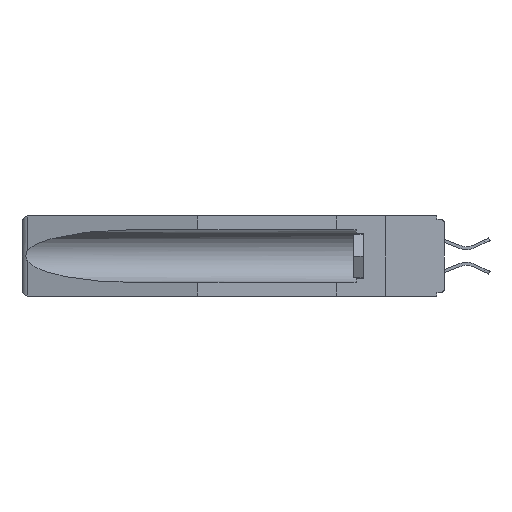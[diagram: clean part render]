
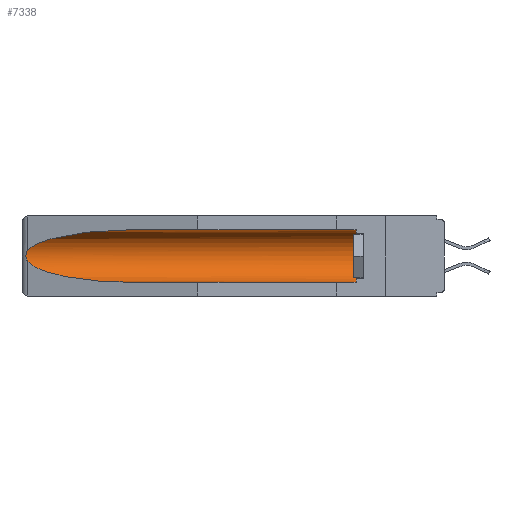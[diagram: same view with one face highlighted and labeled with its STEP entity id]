
A CAD part, left-side view. The second image highlights one B-rep face of the part: STEP entity #7338.
In plain terms, the highlighted cylindrical face has radius 2.857 mm (diameter 5.715 mm), a partial arc.
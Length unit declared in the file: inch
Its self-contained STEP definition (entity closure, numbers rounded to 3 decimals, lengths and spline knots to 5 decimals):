
#56 = LINE ( 'NONE', #18572, #3285 ) ;
#60 = VERTEX_POINT ( 'NONE', #5530 ) ;
#627 = CARTESIAN_POINT ( 'NONE',  ( 0.26537, 1.52718, -0.19328 ) ) ;
#796 = CARTESIAN_POINT ( 'NONE',  ( 0.155, 0.126, -0.1715 ) ) ;
#917 = DIRECTION ( 'NONE',  ( 0., -1., 0. ) ) ;
#1253 = DIRECTION ( 'NONE',  ( 0., 1., 0. ) ) ;
#1864 = EDGE_CURVE ( 'NONE', #13135, #60, #2921, .T. ) ;
#2001 = CARTESIAN_POINT ( 'NONE',  ( 0.26537, 1.52718, -0.19328 ) ) ;
#2046 = CARTESIAN_POINT ( 'NONE',  ( 0.26654, 1.53092, -0.15636 ) ) ;
#2112 = CARTESIAN_POINT ( 'NONE',  ( 0.2675, 1.53308, -0.16763 ) ) ;
#2241 = EDGE_CURVE ( 'NONE', #7680, #8385, #7326, .T. ) ;
#2427 = ORIENTED_EDGE ( 'NONE', *, *, #5106, .T. ) ;
#2921 = CIRCLE ( 'NONE', #15140, 0.1125 ) ;
#3285 = VECTOR ( 'NONE', #14183, 39.37008 ) ;
#3490 = DIRECTION ( 'NONE',  ( 0., 1., 0. ) ) ;
#3847 =( BOUNDED_CURVE ( )  B_SPLINE_CURVE ( 3, ( #2001, #13732, #15233, #9696 ),
 .UNSPECIFIED., .F., .T. ) 
 B_SPLINE_CURVE_WITH_KNOTS ( ( 4, 4 ),
 ( 0.1948, 1.5708 ),
 .UNSPECIFIED. ) 
 CURVE ( )  GEOMETRIC_REPRESENTATION_ITEM ( )  RATIONAL_B_SPLINE_CURVE ( ( 1., 0.848, 0.848, 1. ) ) 
 REPRESENTATION_ITEM ( '' )  );
#4077 = ORIENTED_EDGE ( 'NONE', *, *, #1864, .T. ) ;
#4261 = FACE_OUTER_BOUND ( 'NONE', #14639, .T. ) ;
#4704 = CARTESIAN_POINT ( 'NONE',  ( 0.26537, 1.52718, -0.14972 ) ) ;
#4913 = DIRECTION ( 'NONE',  ( 0., 0., 1. ) ) ;
#5028 = CARTESIAN_POINT ( 'NONE',  ( 0.26537, 1.52718, -0.14972 ) ) ;
#5106 = EDGE_CURVE ( 'NONE', #8385, #9760, #3847, .T. ) ;
#5530 = CARTESIAN_POINT ( 'NONE',  ( 0.155, 0.126, -0.059 ) ) ;
#5545 = CARTESIAN_POINT ( 'NONE',  ( 0.155, 1.07973, -0.059 ) ) ;
#6347 = CYLINDRICAL_SURFACE ( 'NONE', #16453, 0.1125 ) ;
#6887 = ORIENTED_EDGE ( 'NONE', *, *, #7996, .T. ) ;
#6952 = ORIENTED_EDGE ( 'NONE', *, *, #2241, .T. ) ;
#7004 = ORIENTED_EDGE ( 'NONE', *, *, #11708, .T. ) ;
#7242 = CARTESIAN_POINT ( 'NONE',  ( 0.155, 1.07973, -0.284 ) ) ;
#7326 = B_SPLINE_CURVE_WITH_KNOTS ( 'NONE', 3,
 ( #5028, #18506, #2046, #9551, #2112, #17113, #9617, #13848, #13915, #627 ),
 .UNSPECIFIED., .F., .F.,
 ( 4, 2, 2, 2, 4 ),
 ( 0., 0.00029, 0.00058, 0.00087, 0.00117 ),
 .UNSPECIFIED. ) ;
#7338 = ADVANCED_FACE ( 'NONE', ( #4261 ), #6347, .F. ) ;
#7397 = CARTESIAN_POINT ( 'NONE',  ( 0.155, 1.07973, -0.059 ) ) ;
#7680 = VERTEX_POINT ( 'NONE', #9744 ) ;
#7996 = EDGE_CURVE ( 'NONE', #60, #13710, #56, .T. ) ;
#8385 = VERTEX_POINT ( 'NONE', #12537 ) ;
#8836 = EDGE_CURVE ( 'NONE', #13135, #9760, #16421, .T. ) ;
#9551 = CARTESIAN_POINT ( 'NONE',  ( 0.2673, 1.5327, -0.16383 ) ) ;
#9617 = CARTESIAN_POINT ( 'NONE',  ( 0.2673, 1.53269, -0.17917 ) ) ;
#9696 = CARTESIAN_POINT ( 'NONE',  ( 0.155, 1.07973, -0.284 ) ) ;
#9744 = CARTESIAN_POINT ( 'NONE',  ( 0.26537, 1.52718, -0.14972 ) ) ;
#9760 = VERTEX_POINT ( 'NONE', #7242 ) ;
#10126 = CARTESIAN_POINT ( 'NONE',  ( 0.155, -0.30754, -0.284 ) ) ;
#10674 = CARTESIAN_POINT ( 'NONE',  ( 0.25451, 1.48313, -0.09465 ) ) ;
#11708 = EDGE_CURVE ( 'NONE', #13710, #7680, #12926, .T. ) ;
#11805 = CARTESIAN_POINT ( 'NONE',  ( 0.21114, 1.30732, -0.059 ) ) ;
#12456 = VECTOR ( 'NONE', #1253, 39.37008 ) ;
#12537 = CARTESIAN_POINT ( 'NONE',  ( 0.26537, 1.52718, -0.19328 ) ) ;
#12926 =( BOUNDED_CURVE ( )  B_SPLINE_CURVE ( 3, ( #5545, #11805, #10674, #4704 ),
 .UNSPECIFIED., .F., .F. ) 
 B_SPLINE_CURVE_WITH_KNOTS ( ( 4, 4 ),
 ( 4.71239, 6.08839 ),
 .UNSPECIFIED. ) 
 CURVE ( )  GEOMETRIC_REPRESENTATION_ITEM ( )  RATIONAL_B_SPLINE_CURVE ( ( 1., 0.848, 0.848, 1. ) ) 
 REPRESENTATION_ITEM ( '' )  );
#13135 = VERTEX_POINT ( 'NONE', #17829 ) ;
#13360 = ORIENTED_EDGE ( 'NONE', *, *, #8836, .F. ) ;
#13710 = VERTEX_POINT ( 'NONE', #7397 ) ;
#13732 = CARTESIAN_POINT ( 'NONE',  ( 0.25451, 1.48313, -0.24835 ) ) ;
#13848 = CARTESIAN_POINT ( 'NONE',  ( 0.26655, 1.53094, -0.18657 ) ) ;
#13915 = CARTESIAN_POINT ( 'NONE',  ( 0.26597, 1.5296, -0.19026 ) ) ;
#14183 = DIRECTION ( 'NONE',  ( 0., 1., 0. ) ) ;
#14639 = EDGE_LOOP ( 'NONE', ( #7004, #6952, #2427, #13360, #4077, #6887 ) ) ;
#15140 = AXIS2_PLACEMENT_3D ( 'NONE', #796, #917, #15777 ) ;
#15233 = CARTESIAN_POINT ( 'NONE',  ( 0.21114, 1.30732, -0.284 ) ) ;
#15777 = DIRECTION ( 'NONE',  ( 0., 0., 1. ) ) ;
#16421 = LINE ( 'NONE', #10126, #12456 ) ;
#16453 = AXIS2_PLACEMENT_3D ( 'NONE', #18107, #3490, #4913 ) ;
#17113 = CARTESIAN_POINT ( 'NONE',  ( 0.2675, 1.53308, -0.17534 ) ) ;
#17829 = CARTESIAN_POINT ( 'NONE',  ( 0.155, 0.126, -0.284 ) ) ;
#18107 = CARTESIAN_POINT ( 'NONE',  ( 0.155, -0.30754, -0.1715 ) ) ;
#18506 = CARTESIAN_POINT ( 'NONE',  ( 0.26597, 1.52961, -0.15275 ) ) ;
#18572 = CARTESIAN_POINT ( 'NONE',  ( 0.155, -0.30754, -0.059 ) ) ;
